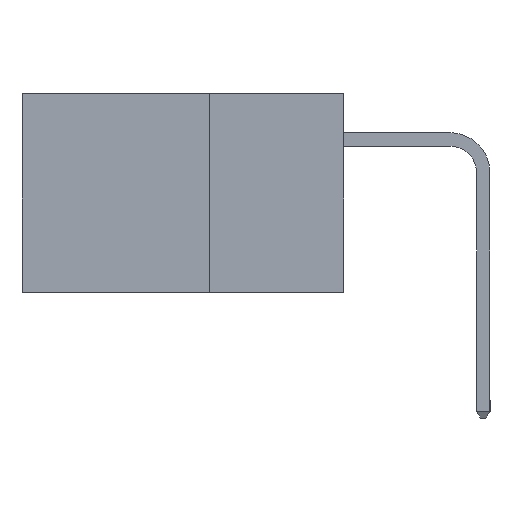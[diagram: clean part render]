
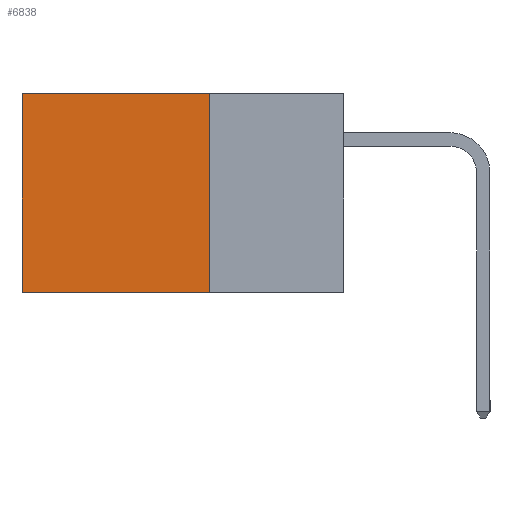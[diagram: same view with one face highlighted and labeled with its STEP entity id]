
A CAD part, left-side view. The second image highlights one B-rep face of the part: STEP entity #6838.
In plain terms, the highlighted planar face has unit normal (-1, 0, 0).
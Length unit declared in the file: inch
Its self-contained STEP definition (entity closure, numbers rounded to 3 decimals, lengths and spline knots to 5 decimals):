
#119 = EDGE_LOOP ( 'NONE', ( #11958, #11913, #3613, #2473 ) ) ;
#268 = CARTESIAN_POINT ( 'NONE',  ( 0.2615, 0.25, -0.37 ) ) ;
#289 = LINE ( 'NONE', #7297, #11611 ) ;
#736 = CARTESIAN_POINT ( 'NONE',  ( 0.2615, 0.6, 0. ) ) ;
#984 = CARTESIAN_POINT ( 'NONE',  ( 0.2615, 0.25, 0. ) ) ;
#1258 = EDGE_CURVE ( 'NONE', #6571, #13439, #12497, .T. ) ;
#2253 = DIRECTION ( 'NONE',  ( 0., 0., -1. ) ) ;
#2473 = ORIENTED_EDGE ( 'NONE', *, *, #9844, .T. ) ;
#3058 = VECTOR ( 'NONE', #2253, 39.37008 ) ;
#3574 = EDGE_CURVE ( 'NONE', #6334, #6571, #4306, .T. ) ;
#3613 = ORIENTED_EDGE ( 'NONE', *, *, #3574, .F. ) ;
#4306 = LINE ( 'NONE', #13695, #10152 ) ;
#4628 = DIRECTION ( 'NONE',  ( 0., 0., -1. ) ) ;
#5141 = LINE ( 'NONE', #9927, #3058 ) ;
#5341 = EDGE_CURVE ( 'NONE', #12308, #13439, #5141, .T. ) ;
#5368 = CARTESIAN_POINT ( 'NONE',  ( 0.2615, 0.6, -0.37 ) ) ;
#6334 = VERTEX_POINT ( 'NONE', #984 ) ;
#6571 = VERTEX_POINT ( 'NONE', #8920 ) ;
#6837 = VECTOR ( 'NONE', #6860, 39.37008 ) ;
#6838 = ADVANCED_FACE ( 'NONE', ( #7540 ), #7948, .F. ) ;
#6860 = DIRECTION ( 'NONE',  ( 0., 1., 0. ) ) ;
#7297 = CARTESIAN_POINT ( 'NONE',  ( 0.2615, 0.25, 0. ) ) ;
#7540 = FACE_OUTER_BOUND ( 'NONE', #119, .T. ) ;
#7948 = PLANE ( 'NONE',  #8300 ) ;
#8300 = AXIS2_PLACEMENT_3D ( 'NONE', #268, #8855, #4628 ) ;
#8855 = DIRECTION ( 'NONE',  ( 1., 0., 0. ) ) ;
#8920 = CARTESIAN_POINT ( 'NONE',  ( 0.2615, 0.25, -0.37 ) ) ;
#9009 = CARTESIAN_POINT ( 'NONE',  ( 0.2615, 0.25, -0.37 ) ) ;
#9844 = EDGE_CURVE ( 'NONE', #6334, #12308, #289, .T. ) ;
#9927 = CARTESIAN_POINT ( 'NONE',  ( 0.2615, 0.6, -0.37 ) ) ;
#10152 = VECTOR ( 'NONE', #10467, 39.37008 ) ;
#10467 = DIRECTION ( 'NONE',  ( 0., 0., -1. ) ) ;
#11611 = VECTOR ( 'NONE', #12588, 39.37008 ) ;
#11913 = ORIENTED_EDGE ( 'NONE', *, *, #1258, .F. ) ;
#11958 = ORIENTED_EDGE ( 'NONE', *, *, #5341, .T. ) ;
#12308 = VERTEX_POINT ( 'NONE', #736 ) ;
#12497 = LINE ( 'NONE', #9009, #6837 ) ;
#12588 = DIRECTION ( 'NONE',  ( 0., 1., 0. ) ) ;
#13439 = VERTEX_POINT ( 'NONE', #5368 ) ;
#13695 = CARTESIAN_POINT ( 'NONE',  ( 0.2615, 0.25, -0.37 ) ) ;
